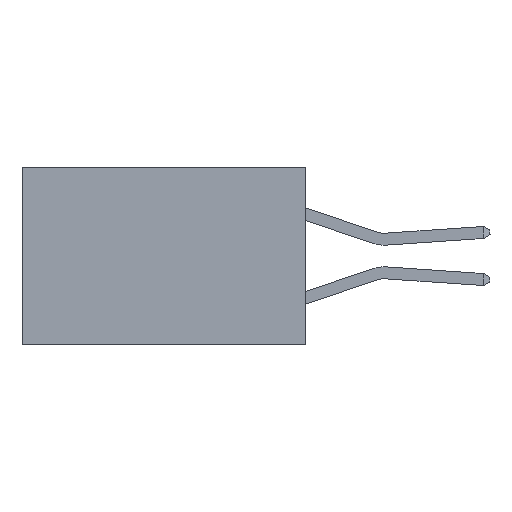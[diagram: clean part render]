
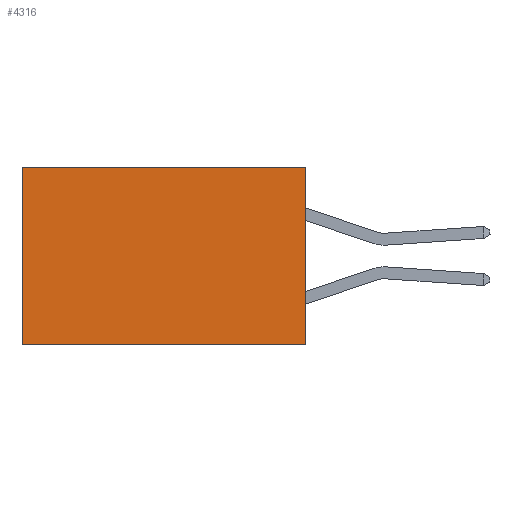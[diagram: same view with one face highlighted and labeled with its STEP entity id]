
A CAD part, left-side view. The second image highlights one B-rep face of the part: STEP entity #4316.
In plain terms, the highlighted planar face has unit normal (-1, 0, 0).
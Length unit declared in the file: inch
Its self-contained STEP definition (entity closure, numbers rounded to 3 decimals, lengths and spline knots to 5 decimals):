
#572 = LINE ( 'NONE', #11608, #9526 ) ;
#894 = FACE_OUTER_BOUND ( 'NONE', #5845, .T. ) ;
#1777 = VERTEX_POINT ( 'NONE', #2899 ) ;
#1811 = VERTEX_POINT ( 'NONE', #12439 ) ;
#1853 = LINE ( 'NONE', #10316, #13311 ) ;
#2187 = VECTOR ( 'NONE', #12650, 39.37008 ) ;
#2458 = ORIENTED_EDGE ( 'NONE', *, *, #3189, .F. ) ;
#2899 = CARTESIAN_POINT ( 'NONE',  ( 0.277, 0., -0.37 ) ) ;
#3084 = EDGE_CURVE ( 'NONE', #1777, #1811, #572, .T. ) ;
#3189 = EDGE_CURVE ( 'NONE', #6541, #1777, #1853, .T. ) ;
#3725 = DIRECTION ( 'NONE',  ( 0., 0., -1. ) ) ;
#4207 = EDGE_CURVE ( 'NONE', #7028, #1811, #11534, .T. ) ;
#4316 = ADVANCED_FACE ( 'NONE', ( #894 ), #14067, .F. ) ;
#4432 = EDGE_CURVE ( 'NONE', #6541, #7028, #5566, .T. ) ;
#5192 = CARTESIAN_POINT ( 'NONE',  ( 0.277, 0.59, -0.37 ) ) ;
#5566 = LINE ( 'NONE', #12751, #2187 ) ;
#5845 = EDGE_LOOP ( 'NONE', ( #11213, #9374, #2458, #8404 ) ) ;
#6541 = VERTEX_POINT ( 'NONE', #12709 ) ;
#7028 = VERTEX_POINT ( 'NONE', #13686 ) ;
#8404 = ORIENTED_EDGE ( 'NONE', *, *, #4432, .T. ) ;
#8687 = VECTOR ( 'NONE', #3725, 39.37008 ) ;
#9374 = ORIENTED_EDGE ( 'NONE', *, *, #3084, .F. ) ;
#9526 = VECTOR ( 'NONE', #12157, 39.37008 ) ;
#10316 = CARTESIAN_POINT ( 'NONE',  ( 0.277, 0., -0.37 ) ) ;
#10334 = DIRECTION ( 'NONE',  ( 0., 0., -1. ) ) ;
#11213 = ORIENTED_EDGE ( 'NONE', *, *, #4207, .T. ) ;
#11534 = LINE ( 'NONE', #5192, #8687 ) ;
#11608 = CARTESIAN_POINT ( 'NONE',  ( 0.277, 0., -0.37 ) ) ;
#11920 = AXIS2_PLACEMENT_3D ( 'NONE', #14208, #14044, #14042 ) ;
#12157 = DIRECTION ( 'NONE',  ( 0., 1., 0. ) ) ;
#12439 = CARTESIAN_POINT ( 'NONE',  ( 0.277, 0.59, -0.37 ) ) ;
#12650 = DIRECTION ( 'NONE',  ( 0., 1., 0. ) ) ;
#12709 = CARTESIAN_POINT ( 'NONE',  ( 0.277, 0., 0. ) ) ;
#12751 = CARTESIAN_POINT ( 'NONE',  ( 0.277, 0., 0. ) ) ;
#13311 = VECTOR ( 'NONE', #10334, 39.37008 ) ;
#13686 = CARTESIAN_POINT ( 'NONE',  ( 0.277, 0.59, 0. ) ) ;
#14042 = DIRECTION ( 'NONE',  ( 0., 0., -1. ) ) ;
#14044 = DIRECTION ( 'NONE',  ( 1., 0., 0. ) ) ;
#14067 = PLANE ( 'NONE',  #11920 ) ;
#14208 = CARTESIAN_POINT ( 'NONE',  ( 0.277, 0., -0.37 ) ) ;
